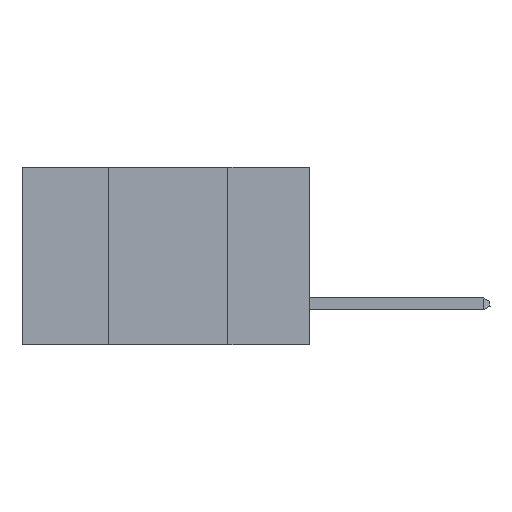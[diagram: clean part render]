
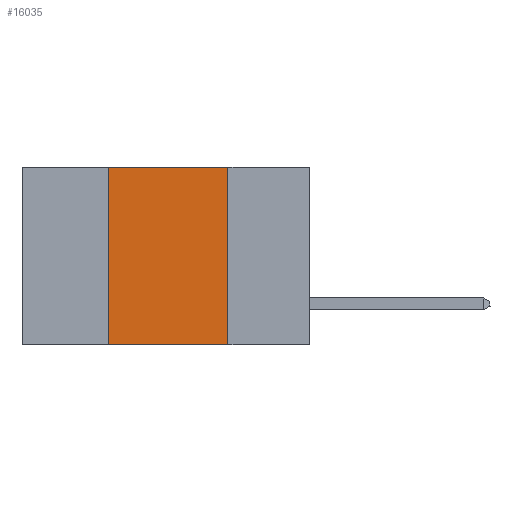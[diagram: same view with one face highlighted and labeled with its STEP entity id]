
A CAD part, left-side view. The second image highlights one B-rep face of the part: STEP entity #16035.
In plain terms, the highlighted planar face has unit normal (-1, 0, 0).
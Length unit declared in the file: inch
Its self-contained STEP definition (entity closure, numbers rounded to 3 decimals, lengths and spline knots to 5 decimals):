
#467 = ORIENTED_EDGE ( 'NONE', *, *, #11295, .F. ) ;
#620 = CARTESIAN_POINT ( 'NONE',  ( 0., 0.6, 0. ) ) ;
#783 = VERTEX_POINT ( 'NONE', #9451 ) ;
#895 = DIRECTION ( 'NONE',  ( 0., -1., 0. ) ) ;
#1457 = VERTEX_POINT ( 'NONE', #14614 ) ;
#2715 = LINE ( 'NONE', #14855, #6400 ) ;
#2775 = ORIENTED_EDGE ( 'NONE', *, *, #3046, .F. ) ;
#2979 = DIRECTION ( 'NONE',  ( 0., 0., -1. ) ) ;
#3046 = EDGE_CURVE ( 'NONE', #9201, #7765, #16480, .T. ) ;
#3231 = LINE ( 'NONE', #7423, #4662 ) ;
#4381 = CARTESIAN_POINT ( 'NONE',  ( 0., 0.42, -0.37 ) ) ;
#4662 = VECTOR ( 'NONE', #895, 39.37008 ) ;
#4664 = DIRECTION ( 'NONE',  ( 0., 0., -1. ) ) ;
#6359 = EDGE_LOOP ( 'NONE', ( #11127, #467, #2775, #9315 ) ) ;
#6400 = VECTOR ( 'NONE', #14738, 39.37008 ) ;
#7423 = CARTESIAN_POINT ( 'NONE',  ( 0., 0.6, -0.37 ) ) ;
#7538 = VECTOR ( 'NONE', #2979, 39.37008 ) ;
#7765 = VERTEX_POINT ( 'NONE', #14864 ) ;
#8453 = FACE_OUTER_BOUND ( 'NONE', #6359, .T. ) ;
#9201 = VERTEX_POINT ( 'NONE', #4381 ) ;
#9315 = ORIENTED_EDGE ( 'NONE', *, *, #13924, .T. ) ;
#9451 = CARTESIAN_POINT ( 'NONE',  ( 0., 0.17, -0.37 ) ) ;
#9927 = VECTOR ( 'NONE', #9933, 39.37008 ) ;
#9933 = DIRECTION ( 'NONE',  ( 0., 0., 1. ) ) ;
#10784 = CARTESIAN_POINT ( 'NONE',  ( 0., 0.17, 0. ) ) ;
#11127 = ORIENTED_EDGE ( 'NONE', *, *, #13077, .F. ) ;
#11295 = EDGE_CURVE ( 'NONE', #7765, #1457, #2715, .T. ) ;
#11436 = LINE ( 'NONE', #10784, #7538 ) ;
#12336 = DIRECTION ( 'NONE',  ( 1., 0., 0. ) ) ;
#12393 = PLANE ( 'NONE',  #15748 ) ;
#13077 = EDGE_CURVE ( 'NONE', #1457, #783, #11436, .T. ) ;
#13924 = EDGE_CURVE ( 'NONE', #9201, #783, #3231, .T. ) ;
#14614 = CARTESIAN_POINT ( 'NONE',  ( 0., 0.17, 0. ) ) ;
#14738 = DIRECTION ( 'NONE',  ( 0., -1., 0. ) ) ;
#14855 = CARTESIAN_POINT ( 'NONE',  ( 0., 0.6, 0. ) ) ;
#14864 = CARTESIAN_POINT ( 'NONE',  ( 0., 0.42, 0. ) ) ;
#15748 = AXIS2_PLACEMENT_3D ( 'NONE', #620, #12336, #4664 ) ;
#16035 = ADVANCED_FACE ( 'NONE', ( #8453 ), #12393, .F. ) ;
#16480 = LINE ( 'NONE', #16622, #9927 ) ;
#16622 = CARTESIAN_POINT ( 'NONE',  ( 0., 0.42, 0. ) ) ;
